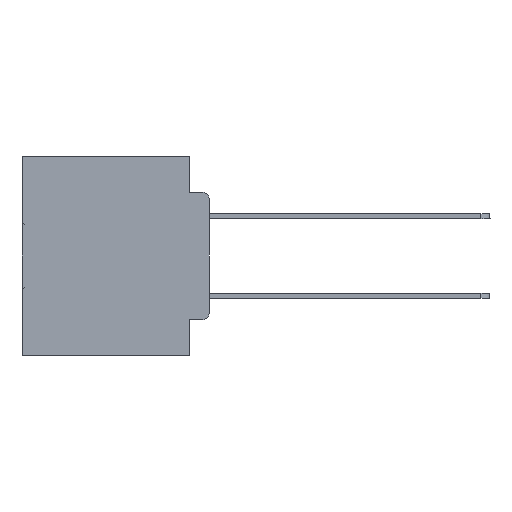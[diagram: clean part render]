
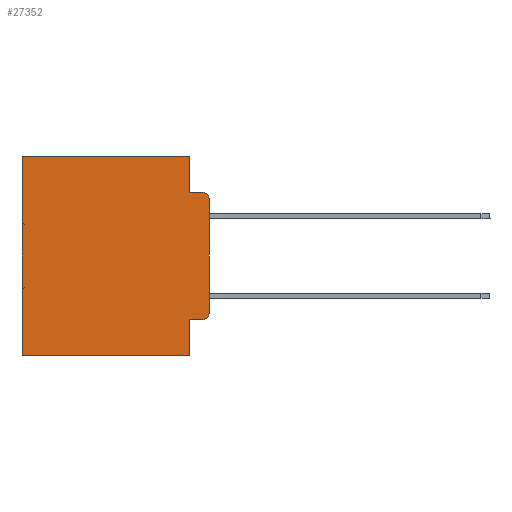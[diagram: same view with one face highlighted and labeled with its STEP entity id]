
A CAD part, left-side view. The second image highlights one B-rep face of the part: STEP entity #27352.
In plain terms, the highlighted planar face has unit normal (-1, 0, 0).
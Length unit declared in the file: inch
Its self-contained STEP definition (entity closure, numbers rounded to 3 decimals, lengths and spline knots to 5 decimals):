
#140 = CIRCLE ( 'NONE', #32251, 0.02 ) ;
#146 = AXIS2_PLACEMENT_3D ( 'NONE', #17348, #34197, #496 ) ;
#481 = LINE ( 'NONE', #19355, #27299 ) ;
#490 = LINE ( 'NONE', #3394, #32535 ) ;
#496 = DIRECTION ( 'NONE',  ( 0., 0., -1. ) ) ;
#518 = CARTESIAN_POINT ( 'NONE',  ( 0.298, 0.02, -0.3915 ) ) ;
#602 = DIRECTION ( 'NONE',  ( 0., 1., 0. ) ) ;
#2845 = ORIENTED_EDGE ( 'NONE', *, *, #17688, .F. ) ;
#3392 = EDGE_CURVE ( 'NONE', #7345, #11280, #140, .T. ) ;
#3394 = CARTESIAN_POINT ( 'NONE',  ( 0.298, 0.051, -0.4115 ) ) ;
#3518 = DIRECTION ( 'NONE',  ( 0., -1., 0. ) ) ;
#3587 = CARTESIAN_POINT ( 'NONE',  ( 0.298, 0., -0.1085 ) ) ;
#3724 = CARTESIAN_POINT ( 'NONE',  ( 0.298, 0.051, 0. ) ) ;
#3846 = CARTESIAN_POINT ( 'NONE',  ( 0.298, 0., 0. ) ) ;
#3886 = VERTEX_POINT ( 'NONE', #23568 ) ;
#3969 = DIRECTION ( 'NONE',  ( 0., 0., -1. ) ) ;
#4603 = LINE ( 'NONE', #5551, #11231 ) ;
#4757 = CIRCLE ( 'NONE', #146, 0.02 ) ;
#4901 = VERTEX_POINT ( 'NONE', #21213 ) ;
#5095 = VERTEX_POINT ( 'NONE', #21951 ) ;
#5415 = ORIENTED_EDGE ( 'NONE', *, *, #6061, .F. ) ;
#5486 = VECTOR ( 'NONE', #14198, 39.37008 ) ;
#5551 = CARTESIAN_POINT ( 'NONE',  ( 0.298, 0., -0.5 ) ) ;
#5569 = CARTESIAN_POINT ( 'NONE',  ( 0.298, 0.051, 0. ) ) ;
#5648 = LINE ( 'NONE', #3724, #20571 ) ;
#6054 = DIRECTION ( 'NONE',  ( 0., -1., 0. ) ) ;
#6061 = EDGE_CURVE ( 'NONE', #11285, #11280, #19497, .T. ) ;
#6852 = AXIS2_PLACEMENT_3D ( 'NONE', #3846, #12470, #34835 ) ;
#7234 = LINE ( 'NONE', #28008, #28690 ) ;
#7345 = VERTEX_POINT ( 'NONE', #27515 ) ;
#8665 = ORIENTED_EDGE ( 'NONE', *, *, #16253, .T. ) ;
#9411 = EDGE_CURVE ( 'NONE', #11285, #5095, #4757, .T. ) ;
#10352 = LINE ( 'NONE', #33516, #5486 ) ;
#11231 = VECTOR ( 'NONE', #602, 39.37008 ) ;
#11280 = VERTEX_POINT ( 'NONE', #29425 ) ;
#11285 = VERTEX_POINT ( 'NONE', #3587 ) ;
#11713 = EDGE_CURVE ( 'NONE', #13498, #27013, #4603, .T. ) ;
#12470 = DIRECTION ( 'NONE',  ( 1., 0., 0. ) ) ;
#12861 = ORIENTED_EDGE ( 'NONE', *, *, #3392, .T. ) ;
#13027 = CARTESIAN_POINT ( 'NONE',  ( 0.298, 0.051, -0.5 ) ) ;
#13498 = VERTEX_POINT ( 'NONE', #13027 ) ;
#14198 = DIRECTION ( 'NONE',  ( 0., 0., -1. ) ) ;
#14316 = DIRECTION ( 'NONE',  ( 0., 0., -1. ) ) ;
#14405 = ORIENTED_EDGE ( 'NONE', *, *, #23633, .T. ) ;
#16232 = ORIENTED_EDGE ( 'NONE', *, *, #11713, .F. ) ;
#16253 = EDGE_CURVE ( 'NONE', #4901, #7345, #490, .T. ) ;
#17348 = CARTESIAN_POINT ( 'NONE',  ( 0.298, 0.02, -0.1085 ) ) ;
#17688 = EDGE_CURVE ( 'NONE', #4901, #13498, #35080, .T. ) ;
#17724 = VECTOR ( 'NONE', #23147, 39.37008 ) ;
#19355 = CARTESIAN_POINT ( 'NONE',  ( 0.298, 0., 0. ) ) ;
#19497 = LINE ( 'NONE', #22789, #17724 ) ;
#19773 = ORIENTED_EDGE ( 'NONE', *, *, #27486, .F. ) ;
#20517 = ORIENTED_EDGE ( 'NONE', *, *, #25261, .T. ) ;
#20571 = VECTOR ( 'NONE', #3969, 39.37008 ) ;
#21213 = CARTESIAN_POINT ( 'NONE',  ( 0.298, 0.051, -0.4115 ) ) ;
#21951 = CARTESIAN_POINT ( 'NONE',  ( 0.298, 0.02, -0.0885 ) ) ;
#22789 = CARTESIAN_POINT ( 'NONE',  ( 0.298, 0., 0. ) ) ;
#23147 = DIRECTION ( 'NONE',  ( 0., 0., -1. ) ) ;
#23422 = ORIENTED_EDGE ( 'NONE', *, *, #30362, .F. ) ;
#23568 = CARTESIAN_POINT ( 'NONE',  ( 0.298, 0.051, -0.0885 ) ) ;
#23633 = EDGE_CURVE ( 'NONE', #24502, #27013, #10352, .T. ) ;
#24502 = VERTEX_POINT ( 'NONE', #34654 ) ;
#24596 = CARTESIAN_POINT ( 'NONE',  ( 0.298, 0.051, 0. ) ) ;
#25261 = EDGE_CURVE ( 'NONE', #30907, #24502, #481, .T. ) ;
#26448 = ORIENTED_EDGE ( 'NONE', *, *, #9411, .T. ) ;
#27013 = VERTEX_POINT ( 'NONE', #27073 ) ;
#27073 = CARTESIAN_POINT ( 'NONE',  ( 0.298, 0.473, -0.5 ) ) ;
#27299 = VECTOR ( 'NONE', #35591, 39.37008 ) ;
#27352 = ADVANCED_FACE ( 'NONE', ( #29358 ), #32044, .F. ) ;
#27486 = EDGE_CURVE ( 'NONE', #30907, #3886, #5648, .T. ) ;
#27515 = CARTESIAN_POINT ( 'NONE',  ( 0.298, 0.02, -0.4115 ) ) ;
#27891 = DIRECTION ( 'NONE',  ( 0., 0., -1. ) ) ;
#27937 = EDGE_LOOP ( 'NONE', ( #5415, #26448, #23422, #19773, #20517, #14405, #16232, #2845, #8665, #12861 ) ) ;
#28008 = CARTESIAN_POINT ( 'NONE',  ( 0.298, 0.051, -0.0885 ) ) ;
#28365 = DIRECTION ( 'NONE',  ( -1., 0., 0. ) ) ;
#28690 = VECTOR ( 'NONE', #6054, 39.37008 ) ;
#29358 = FACE_OUTER_BOUND ( 'NONE', #27937, .T. ) ;
#29425 = CARTESIAN_POINT ( 'NONE',  ( 0.298, 0., -0.3915 ) ) ;
#30362 = EDGE_CURVE ( 'NONE', #3886, #5095, #7234, .T. ) ;
#30907 = VERTEX_POINT ( 'NONE', #24596 ) ;
#32044 = PLANE ( 'NONE',  #6852 ) ;
#32045 = VECTOR ( 'NONE', #27891, 39.37008 ) ;
#32251 = AXIS2_PLACEMENT_3D ( 'NONE', #518, #28365, #14316 ) ;
#32535 = VECTOR ( 'NONE', #3518, 39.37008 ) ;
#33516 = CARTESIAN_POINT ( 'NONE',  ( 0.298, 0.473, 0. ) ) ;
#34197 = DIRECTION ( 'NONE',  ( -1., 0., 0. ) ) ;
#34654 = CARTESIAN_POINT ( 'NONE',  ( 0.298, 0.473, 0. ) ) ;
#34835 = DIRECTION ( 'NONE',  ( 0., 0., -1. ) ) ;
#35080 = LINE ( 'NONE', #5569, #32045 ) ;
#35591 = DIRECTION ( 'NONE',  ( 0., 1., 0. ) ) ;
